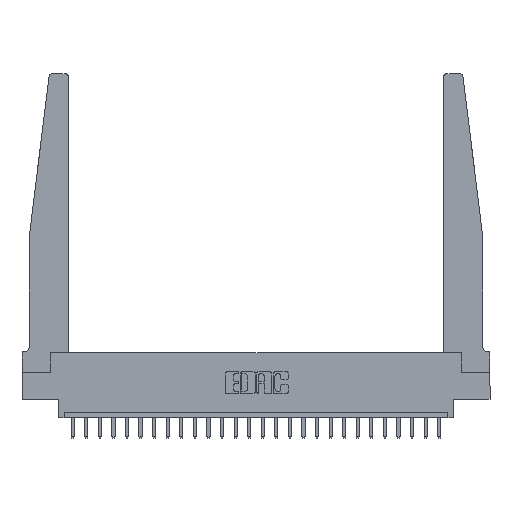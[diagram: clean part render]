
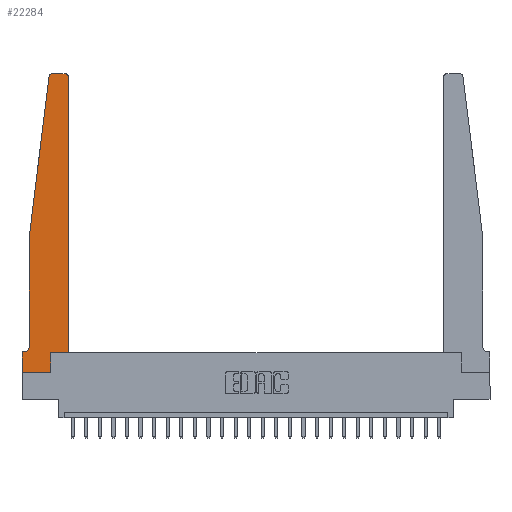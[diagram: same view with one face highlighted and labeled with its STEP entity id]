
A CAD part, top view. The second image highlights one B-rep face of the part: STEP entity #22284.
In plain terms, the highlighted planar face has unit normal (0, 0, 1).
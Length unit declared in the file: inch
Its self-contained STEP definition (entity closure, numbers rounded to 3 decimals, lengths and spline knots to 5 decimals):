
#166 = ORIENTED_EDGE ( 'NONE', *, *, #17380, .T. ) ;
#232 = ORIENTED_EDGE ( 'NONE', *, *, #11201, .T. ) ;
#425 = EDGE_CURVE ( 'NONE', #1578, #13352, #12317, .T. ) ;
#435 = AXIS2_PLACEMENT_3D ( 'NONE', #21554, #23351, #8402 ) ;
#882 = EDGE_CURVE ( 'NONE', #24165, #14620, #18742, .T. ) ;
#1225 = DIRECTION ( 'NONE',  ( 0., 1., 0. ) ) ;
#1243 = LINE ( 'NONE', #11297, #3324 ) ;
#1578 = VERTEX_POINT ( 'NONE', #13642 ) ;
#1735 = DIRECTION ( 'NONE',  ( 0., 0., 1. ) ) ;
#2359 = VECTOR ( 'NONE', #6869, 39.37008 ) ;
#2470 = CIRCLE ( 'NONE', #435, 0.05 ) ;
#2958 = VERTEX_POINT ( 'NONE', #17674 ) ;
#3324 = VECTOR ( 'NONE', #11366, 39.37008 ) ;
#3819 = LINE ( 'NONE', #4571, #24034 ) ;
#4201 = ORIENTED_EDGE ( 'NONE', *, *, #22100, .T. ) ;
#4495 = VERTEX_POINT ( 'NONE', #14931 ) ;
#4571 = CARTESIAN_POINT ( 'NONE',  ( 0.065, 1.25, 0.37 ) ) ;
#4773 = ORIENTED_EDGE ( 'NONE', *, *, #9690, .T. ) ;
#4815 = CARTESIAN_POINT ( 'NONE',  ( 0.065, 0.2375, 0.37 ) ) ;
#4835 = CARTESIAN_POINT ( 'NONE',  ( 0., 0., 0.37 ) ) ;
#4914 = CARTESIAN_POINT ( 'NONE',  ( 0., 0.1875, 0.37 ) ) ;
#4953 = DIRECTION ( 'NONE',  ( 1., 0., 0. ) ) ;
#6274 = EDGE_CURVE ( 'NONE', #24096, #15746, #8857, .T. ) ;
#6292 = DIRECTION ( 'NONE',  ( -1., 0., 0. ) ) ;
#6718 = DIRECTION ( 'NONE',  ( 1., 0., 0. ) ) ;
#6869 = DIRECTION ( 'NONE',  ( 0., 1., 0. ) ) ;
#7436 = CARTESIAN_POINT ( 'NONE',  ( 0.015, 0.1875, 0.37 ) ) ;
#7627 = EDGE_CURVE ( 'NONE', #2958, #19219, #21154, .T. ) ;
#7911 = CARTESIAN_POINT ( 'NONE',  ( 0.425, 2.72, 0.37 ) ) ;
#8328 = DIRECTION ( 'NONE',  ( -0.122, -0.992, 0. ) ) ;
#8402 = DIRECTION ( 'NONE',  ( -1., 0., 0. ) ) ;
#8499 = ORIENTED_EDGE ( 'NONE', *, *, #15805, .T. ) ;
#8857 = LINE ( 'NONE', #15697, #11475 ) ;
#9690 = EDGE_CURVE ( 'NONE', #14516, #1578, #15836, .T. ) ;
#10170 = VERTEX_POINT ( 'NONE', #17776 ) ;
#10393 = CARTESIAN_POINT ( 'NONE',  ( 0.27653, 2.75, 0.37 ) ) ;
#10400 = CARTESIAN_POINT ( 'NONE',  ( 0.27653, 2.72, 0.37 ) ) ;
#10423 = CARTESIAN_POINT ( 'NONE',  ( 0.425, 0.18, 0.37 ) ) ;
#11135 = VECTOR ( 'NONE', #22470, 39.37008 ) ;
#11201 = EDGE_CURVE ( 'NONE', #15746, #14516, #13073, .T. ) ;
#11297 = CARTESIAN_POINT ( 'NONE',  ( 0.065, 1.25, 0.37 ) ) ;
#11366 = DIRECTION ( 'NONE',  ( 0., -1., 0. ) ) ;
#11475 = VECTOR ( 'NONE', #6292, 39.37008 ) ;
#12317 = LINE ( 'NONE', #16358, #2359 ) ;
#12543 = CARTESIAN_POINT ( 'NONE',  ( 0.395, 2.72, 0.37 ) ) ;
#13073 = LINE ( 'NONE', #15155, #19256 ) ;
#13352 = VERTEX_POINT ( 'NONE', #20424 ) ;
#13642 = CARTESIAN_POINT ( 'NONE',  ( 0.2605, 0., 0.37 ) ) ;
#13646 = ORIENTED_EDGE ( 'NONE', *, *, #15064, .T. ) ;
#13757 = CIRCLE ( 'NONE', #15753, 0.03 ) ;
#14201 = LINE ( 'NONE', #15703, #16583 ) ;
#14516 = VERTEX_POINT ( 'NONE', #15609 ) ;
#14620 = VERTEX_POINT ( 'NONE', #10393 ) ;
#14831 = DIRECTION ( 'NONE',  ( 1., 0., 0. ) ) ;
#14860 = CARTESIAN_POINT ( 'NONE',  ( 0.395, 2.75, 0.37 ) ) ;
#14931 = CARTESIAN_POINT ( 'NONE',  ( 0.065, 1.25, 0.37 ) ) ;
#15064 = EDGE_CURVE ( 'NONE', #13352, #2958, #14201, .T. ) ;
#15155 = CARTESIAN_POINT ( 'NONE',  ( 0., 0., 0.37 ) ) ;
#15609 = CARTESIAN_POINT ( 'NONE',  ( 0., 0., 0.37 ) ) ;
#15697 = CARTESIAN_POINT ( 'NONE',  ( 0.065, 0.1875, 0.37 ) ) ;
#15703 = CARTESIAN_POINT ( 'NONE',  ( 0.425, 0.18, 0.37 ) ) ;
#15746 = VERTEX_POINT ( 'NONE', #4914 ) ;
#15753 = AXIS2_PLACEMENT_3D ( 'NONE', #12543, #20254, #4953 ) ;
#15805 = EDGE_CURVE ( 'NONE', #24073, #24096, #2470, .T. ) ;
#15836 = LINE ( 'NONE', #4835, #22847 ) ;
#16109 = ORIENTED_EDGE ( 'NONE', *, *, #17746, .T. ) ;
#16358 = CARTESIAN_POINT ( 'NONE',  ( 0.2605, 0.18, 0.37 ) ) ;
#16583 = VECTOR ( 'NONE', #19617, 39.37008 ) ;
#17380 = EDGE_CURVE ( 'NONE', #14620, #10170, #23216, .T. ) ;
#17655 = VECTOR ( 'NONE', #1225, 39.37008 ) ;
#17674 = CARTESIAN_POINT ( 'NONE',  ( 0.425, 0.18, 0.37 ) ) ;
#17746 = EDGE_CURVE ( 'NONE', #4495, #24073, #1243, .T. ) ;
#17776 = CARTESIAN_POINT ( 'NONE',  ( 0.24675, 2.72367, 0.37 ) ) ;
#18226 = ORIENTED_EDGE ( 'NONE', *, *, #425, .T. ) ;
#18536 = PLANE ( 'NONE',  #22924 ) ;
#18742 = LINE ( 'NONE', #20542, #11135 ) ;
#19118 = ORIENTED_EDGE ( 'NONE', *, *, #882, .T. ) ;
#19219 = VERTEX_POINT ( 'NONE', #7911 ) ;
#19256 = VECTOR ( 'NONE', #20568, 39.37008 ) ;
#19368 = EDGE_CURVE ( 'NONE', #10170, #4495, #3819, .T. ) ;
#19617 = DIRECTION ( 'NONE',  ( 1., 0., 0. ) ) ;
#19915 = ORIENTED_EDGE ( 'NONE', *, *, #19368, .T. ) ;
#20254 = DIRECTION ( 'NONE',  ( 0., 0., 1. ) ) ;
#20424 = CARTESIAN_POINT ( 'NONE',  ( 0.2605, 0.18, 0.37 ) ) ;
#20542 = CARTESIAN_POINT ( 'NONE',  ( 0.25, 2.75, 0.37 ) ) ;
#20568 = DIRECTION ( 'NONE',  ( 0., -1., 0. ) ) ;
#21048 = ORIENTED_EDGE ( 'NONE', *, *, #6274, .T. ) ;
#21154 = LINE ( 'NONE', #10423, #17655 ) ;
#21393 = EDGE_LOOP ( 'NONE', ( #19118, #166, #19915, #16109, #8499, #21048, #232, #4773, #18226, #13646, #24029, #4201 ) ) ;
#21554 = CARTESIAN_POINT ( 'NONE',  ( 0.015, 0.2375, 0.37 ) ) ;
#21667 = FACE_OUTER_BOUND ( 'NONE', #21393, .T. ) ;
#22100 = EDGE_CURVE ( 'NONE', #19219, #24165, #13757, .T. ) ;
#22284 = ADVANCED_FACE ( 'NONE', ( #21667 ), #18536, .T. ) ;
#22470 = DIRECTION ( 'NONE',  ( -1., 0., 0. ) ) ;
#22847 = VECTOR ( 'NONE', #6718, 39.37008 ) ;
#22924 = AXIS2_PLACEMENT_3D ( 'NONE', #24259, #1735, #14831 ) ;
#23216 = CIRCLE ( 'NONE', #23785, 0.03 ) ;
#23351 = DIRECTION ( 'NONE',  ( 0., 0., -1. ) ) ;
#23483 = DIRECTION ( 'NONE',  ( 0., 0., 1. ) ) ;
#23661 = DIRECTION ( 'NONE',  ( 1., 0., 0. ) ) ;
#23785 = AXIS2_PLACEMENT_3D ( 'NONE', #10400, #23483, #23661 ) ;
#24029 = ORIENTED_EDGE ( 'NONE', *, *, #7627, .T. ) ;
#24034 = VECTOR ( 'NONE', #8328, 39.37008 ) ;
#24073 = VERTEX_POINT ( 'NONE', #4815 ) ;
#24096 = VERTEX_POINT ( 'NONE', #7436 ) ;
#24165 = VERTEX_POINT ( 'NONE', #14860 ) ;
#24259 = CARTESIAN_POINT ( 'NONE',  ( 0., 0.1875, 0.37 ) ) ;
